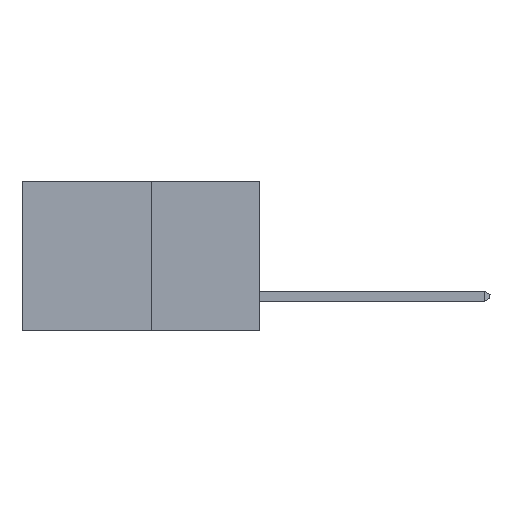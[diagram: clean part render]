
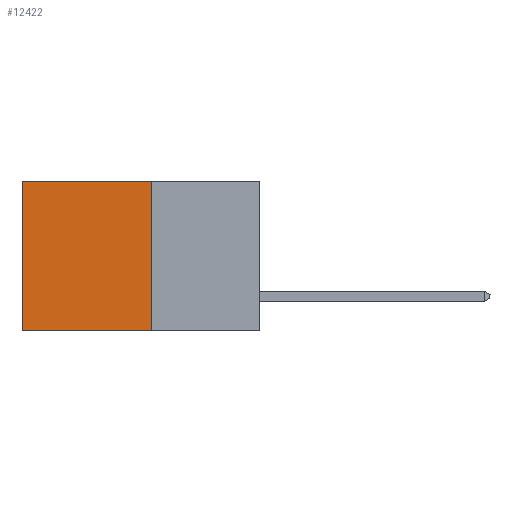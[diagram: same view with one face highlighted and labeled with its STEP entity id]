
A CAD part, left-side view. The second image highlights one B-rep face of the part: STEP entity #12422.
In plain terms, the highlighted planar face has unit normal (-1, 0, 0).
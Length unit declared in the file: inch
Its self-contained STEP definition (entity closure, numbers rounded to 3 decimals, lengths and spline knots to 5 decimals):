
#634 = DIRECTION ( 'NONE',  ( 0., 0., -1. ) ) ;
#831 = LINE ( 'NONE', #14439, #15885 ) ;
#1064 = VECTOR ( 'NONE', #18252, 39.37008 ) ;
#1079 = VECTOR ( 'NONE', #5020, 39.37008 ) ;
#1508 = ORIENTED_EDGE ( 'NONE', *, *, #10017, .T. ) ;
#2277 = AXIS2_PLACEMENT_3D ( 'NONE', #24833, #15463, #3724 ) ;
#2641 = CARTESIAN_POINT ( 'NONE',  ( 0.277, 0.27, -0.37 ) ) ;
#2784 = CARTESIAN_POINT ( 'NONE',  ( 0.277, 0.27, -0.37 ) ) ;
#2873 = CARTESIAN_POINT ( 'NONE',  ( 0.277, 0.27, 0. ) ) ;
#3724 = DIRECTION ( 'NONE',  ( 0., 0., -1. ) ) ;
#4029 = ORIENTED_EDGE ( 'NONE', *, *, #22616, .F. ) ;
#5020 = DIRECTION ( 'NONE',  ( 0., 1., 0. ) ) ;
#5206 = CARTESIAN_POINT ( 'NONE',  ( 0.277, 0.27, 0. ) ) ;
#6325 = LINE ( 'NONE', #2641, #1064 ) ;
#8417 = CARTESIAN_POINT ( 'NONE',  ( 0.277, 0.59, -0.37 ) ) ;
#9464 = FACE_OUTER_BOUND ( 'NONE', #18602, .T. ) ;
#10017 = EDGE_CURVE ( 'NONE', #20873, #10865, #21767, .T. ) ;
#10865 = VERTEX_POINT ( 'NONE', #18771 ) ;
#11716 = LINE ( 'NONE', #21608, #21285 ) ;
#12422 = ADVANCED_FACE ( 'NONE', ( #9464 ), #13546, .F. ) ;
#13546 = PLANE ( 'NONE',  #2277 ) ;
#13842 = EDGE_CURVE ( 'NONE', #18424, #20140, #6325, .T. ) ;
#14439 = CARTESIAN_POINT ( 'NONE',  ( 0.277, 0.59, -0.37 ) ) ;
#15186 = ORIENTED_EDGE ( 'NONE', *, *, #20185, .T. ) ;
#15463 = DIRECTION ( 'NONE',  ( 1., 0., 0. ) ) ;
#15885 = VECTOR ( 'NONE', #634, 39.37008 ) ;
#18252 = DIRECTION ( 'NONE',  ( 0., 1., 0. ) ) ;
#18424 = VERTEX_POINT ( 'NONE', #2784 ) ;
#18602 = EDGE_LOOP ( 'NONE', ( #15186, #24290, #4029, #1508 ) ) ;
#18771 = CARTESIAN_POINT ( 'NONE',  ( 0.277, 0.59, 0. ) ) ;
#20140 = VERTEX_POINT ( 'NONE', #8417 ) ;
#20185 = EDGE_CURVE ( 'NONE', #10865, #20140, #831, .T. ) ;
#20873 = VERTEX_POINT ( 'NONE', #2873 ) ;
#21285 = VECTOR ( 'NONE', #23485, 39.37008 ) ;
#21608 = CARTESIAN_POINT ( 'NONE',  ( 0.277, 0.27, -0.37 ) ) ;
#21767 = LINE ( 'NONE', #5206, #1079 ) ;
#22616 = EDGE_CURVE ( 'NONE', #20873, #18424, #11716, .T. ) ;
#23485 = DIRECTION ( 'NONE',  ( 0., 0., -1. ) ) ;
#24290 = ORIENTED_EDGE ( 'NONE', *, *, #13842, .F. ) ;
#24833 = CARTESIAN_POINT ( 'NONE',  ( 0.277, 0.27, -0.37 ) ) ;
